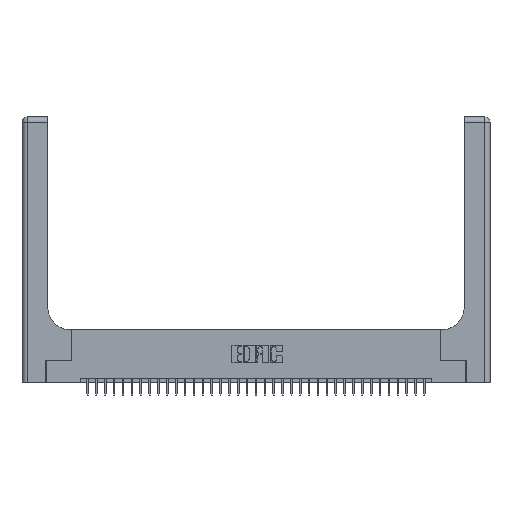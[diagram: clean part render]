
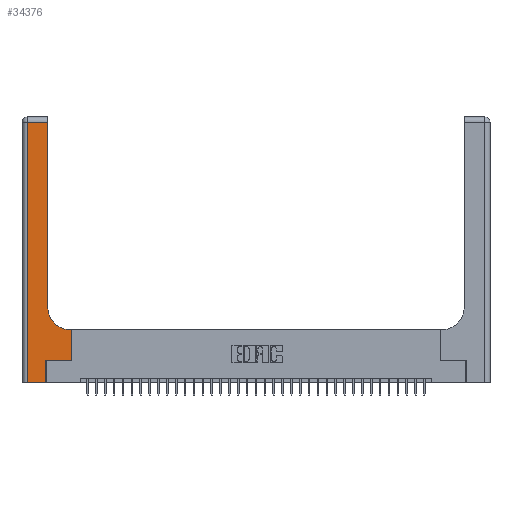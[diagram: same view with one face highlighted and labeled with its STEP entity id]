
A CAD part, top view. The second image highlights one B-rep face of the part: STEP entity #34376.
In plain terms, the highlighted planar face has unit normal (0, 0, 1).
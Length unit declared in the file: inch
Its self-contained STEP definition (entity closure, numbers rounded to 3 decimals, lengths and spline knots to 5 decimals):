
#49 = ORIENTED_EDGE ( 'NONE', *, *, #2175, .T. ) ;
#76 = CARTESIAN_POINT ( 'NONE',  ( 0.5585, 0.25, 0.37 ) ) ;
#874 = LINE ( 'NONE', #23105, #15832 ) ;
#1664 = LINE ( 'NONE', #6463, #9516 ) ;
#2094 = CARTESIAN_POINT ( 'NONE',  ( 0.06, 2.94, 0.37 ) ) ;
#2175 = EDGE_CURVE ( 'NONE', #2342, #23740, #31812, .T. ) ;
#2342 = VERTEX_POINT ( 'NONE', #18439 ) ;
#2471 = VERTEX_POINT ( 'NONE', #16742 ) ;
#4666 = EDGE_CURVE ( 'NONE', #27661, #2471, #36100, .T. ) ;
#5182 = VERTEX_POINT ( 'NONE', #2094 ) ;
#6463 = CARTESIAN_POINT ( 'NONE',  ( 0., 0., 0.37 ) ) ;
#6622 = CARTESIAN_POINT ( 'NONE',  ( 0.2915, 3., 0.37 ) ) ;
#7766 = ORIENTED_EDGE ( 'NONE', *, *, #10469, .T. ) ;
#8192 = VERTEX_POINT ( 'NONE', #31952 ) ;
#8536 = ORIENTED_EDGE ( 'NONE', *, *, #21785, .T. ) ;
#8629 = VERTEX_POINT ( 'NONE', #34295 ) ;
#8948 = CARTESIAN_POINT ( 'NONE',  ( 0., 2.94, 0.37 ) ) ;
#9448 = DIRECTION ( 'NONE',  ( 0., 0., -1. ) ) ;
#9516 = VECTOR ( 'NONE', #15608, 39.37008 ) ;
#10469 = EDGE_CURVE ( 'NONE', #8629, #27661, #23977, .T. ) ;
#10928 = DIRECTION ( 'NONE',  ( 0., 1., 0. ) ) ;
#11125 = LINE ( 'NONE', #11666, #35476 ) ;
#11332 = EDGE_CURVE ( 'NONE', #23740, #17119, #31789, .T. ) ;
#11512 = CARTESIAN_POINT ( 'NONE',  ( 0.5415, 0.85, 0.37 ) ) ;
#11666 = CARTESIAN_POINT ( 'NONE',  ( 0.06, 3., 0.37 ) ) ;
#12029 = PLANE ( 'NONE',  #26071 ) ;
#12078 = CARTESIAN_POINT ( 'NONE',  ( 0.2915, 0.85, 0.37 ) ) ;
#12891 = ORIENTED_EDGE ( 'NONE', *, *, #11332, .T. ) ;
#13377 = CARTESIAN_POINT ( 'NONE',  ( 0.269, 0., 0.37 ) ) ;
#13462 = CARTESIAN_POINT ( 'NONE',  ( 0.2915, 2.94, 0.37 ) ) ;
#14110 = ORIENTED_EDGE ( 'NONE', *, *, #34220, .T. ) ;
#15606 = VECTOR ( 'NONE', #31878, 39.37008 ) ;
#15608 = DIRECTION ( 'NONE',  ( 1., 0., 0. ) ) ;
#15832 = VECTOR ( 'NONE', #28594, 39.37008 ) ;
#16614 = ORIENTED_EDGE ( 'NONE', *, *, #4666, .T. ) ;
#16742 = CARTESIAN_POINT ( 'NONE',  ( 0.5585, 0.6, 0.37 ) ) ;
#16837 = CARTESIAN_POINT ( 'NONE',  ( 0.5585, 0.25, 0.37 ) ) ;
#17069 = VECTOR ( 'NONE', #24806, 39.37008 ) ;
#17119 = VERTEX_POINT ( 'NONE', #13462 ) ;
#17626 = EDGE_CURVE ( 'NONE', #32126, #8629, #30301, .T. ) ;
#17823 = DIRECTION ( 'NONE',  ( 0., 1., 0. ) ) ;
#18425 = VECTOR ( 'NONE', #10928, 39.37008 ) ;
#18439 = CARTESIAN_POINT ( 'NONE',  ( 0.5415, 0.6, 0.37 ) ) ;
#18588 = FACE_OUTER_BOUND ( 'NONE', #23648, .T. ) ;
#19135 = EDGE_CURVE ( 'NONE', #8192, #32126, #1664, .T. ) ;
#21785 = EDGE_CURVE ( 'NONE', #17119, #5182, #31359, .T. ) ;
#23022 = AXIS2_PLACEMENT_3D ( 'NONE', #11512, #9448, #23960 ) ;
#23105 = CARTESIAN_POINT ( 'NONE',  ( 0.2915, 0.6, 0.37 ) ) ;
#23250 = DIRECTION ( 'NONE',  ( 0., 0., -1. ) ) ;
#23648 = EDGE_LOOP ( 'NONE', ( #12891, #8536, #14110, #23708, #24471, #7766, #16614, #29477, #49 ) ) ;
#23708 = ORIENTED_EDGE ( 'NONE', *, *, #19135, .T. ) ;
#23740 = VERTEX_POINT ( 'NONE', #12078 ) ;
#23960 = DIRECTION ( 'NONE',  ( 1., 0., 0. ) ) ;
#23977 = LINE ( 'NONE', #34991, #15606 ) ;
#24061 = CARTESIAN_POINT ( 'NONE',  ( 0.269, 0., 0.37 ) ) ;
#24471 = ORIENTED_EDGE ( 'NONE', *, *, #17626, .T. ) ;
#24806 = DIRECTION ( 'NONE',  ( 0., 1., 0. ) ) ;
#26071 = AXIS2_PLACEMENT_3D ( 'NONE', #29789, #23250, #34441 ) ;
#27661 = VERTEX_POINT ( 'NONE', #16837 ) ;
#28194 = DIRECTION ( 'NONE',  ( 0., -1., 0. ) ) ;
#28563 = VECTOR ( 'NONE', #17823, 39.37008 ) ;
#28594 = DIRECTION ( 'NONE',  ( -1., 0., 0. ) ) ;
#28991 = EDGE_CURVE ( 'NONE', #2471, #2342, #874, .T. ) ;
#29477 = ORIENTED_EDGE ( 'NONE', *, *, #28991, .T. ) ;
#29789 = CARTESIAN_POINT ( 'NONE',  ( 0., 3., 0.37 ) ) ;
#30301 = LINE ( 'NONE', #13377, #17069 ) ;
#31359 = LINE ( 'NONE', #8948, #32606 ) ;
#31789 = LINE ( 'NONE', #6622, #28563 ) ;
#31812 = CIRCLE ( 'NONE', #23022, 0.25 ) ;
#31878 = DIRECTION ( 'NONE',  ( 1., 0., 0. ) ) ;
#31952 = CARTESIAN_POINT ( 'NONE',  ( 0.06, 0., 0.37 ) ) ;
#32126 = VERTEX_POINT ( 'NONE', #24061 ) ;
#32606 = VECTOR ( 'NONE', #34288, 39.37008 ) ;
#34220 = EDGE_CURVE ( 'NONE', #5182, #8192, #11125, .T. ) ;
#34288 = DIRECTION ( 'NONE',  ( -1., 0., 0. ) ) ;
#34295 = CARTESIAN_POINT ( 'NONE',  ( 0.269, 0.25, 0.37 ) ) ;
#34376 = ADVANCED_FACE ( 'NONE', ( #18588 ), #12029, .F. ) ;
#34441 = DIRECTION ( 'NONE',  ( -1., 0., 0. ) ) ;
#34991 = CARTESIAN_POINT ( 'NONE',  ( 0.269, 0.25, 0.37 ) ) ;
#35476 = VECTOR ( 'NONE', #28194, 39.37008 ) ;
#36100 = LINE ( 'NONE', #76, #18425 ) ;
